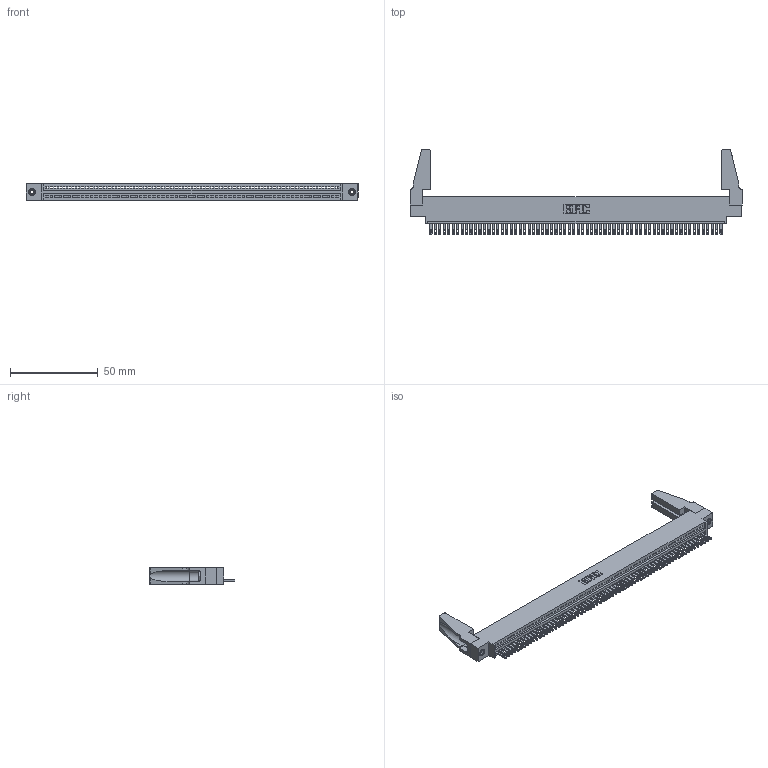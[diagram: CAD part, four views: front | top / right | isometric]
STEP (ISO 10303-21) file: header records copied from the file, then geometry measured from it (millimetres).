
FILE_DESCRIPTION (( 'STEP AP203' ), '1' );
FILE_NAME ('345-066-500-688.STEP', '2019-10-11T19:59:16', ( '' ), ( '' ), 'SwSTEP 2.0', 'SolidWorks 2016', '' );
FILE_SCHEMA (( 'CONFIG_CONTROL_DESIGN' ));
Length unit declared in the file: inch
Products named in the file (5): 345-220-078_345-220-088; 345-066-500-688; 345 Part_0.170 Offset - 0.156 Dia-TH; 345-292-001_345-293-100; 345-250-001_345-250-001-102
Assembly tree (71 placements, depth 2):
  345-066-500-688
    345 Part_0.170 Offset - 0.156 Dia-TH
    345-292-001_345-293-100  x66
    345-250-001_345-250-001-102  x2
    345-220-078_345-220-088  x2
Bounding box: 188.87 x 48.69 x 9.4 mm (x, y, z)
Volume: 21316 mm3; surface area: 27735 mm2
Topology: 71 solids, 71 shells, 3818 faces, 11755 edges, 7826 vertices
Faces by surface type: plane 2400, cylinder 1402, cone 12, torus 4
Entity records: 48652 total; most frequent: CARTESIAN_POINT 8416, ORIENTED_EDGE 8376, DIRECTION 7324, EDGE_CURVE 4188, LINE 3746, VECTOR 3746, VERTEX_POINT 2786, AXIS2_PLACEMENT_3D 1789
